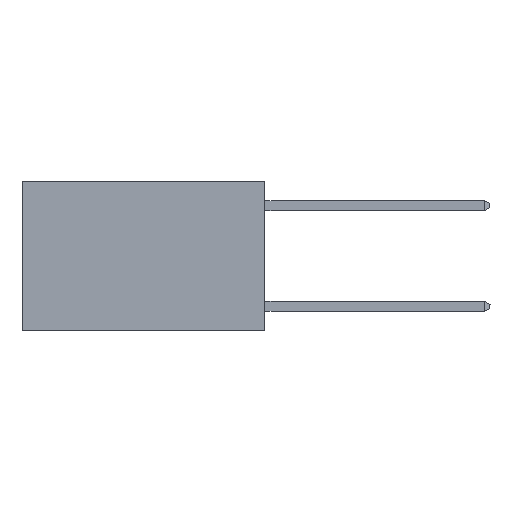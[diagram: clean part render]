
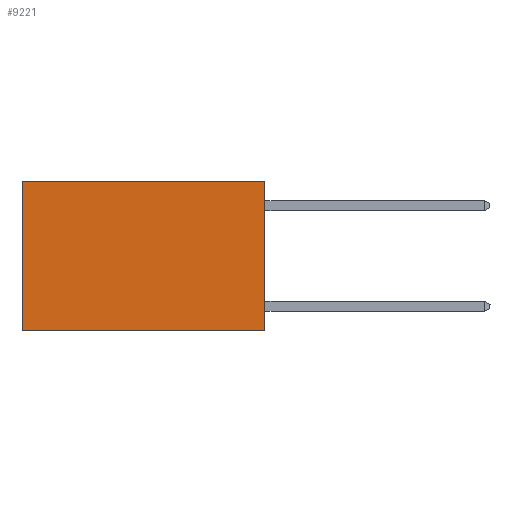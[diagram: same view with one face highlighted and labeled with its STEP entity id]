
A CAD part, left-side view. The second image highlights one B-rep face of the part: STEP entity #9221.
In plain terms, the highlighted planar face has unit normal (-1, 0, 0).
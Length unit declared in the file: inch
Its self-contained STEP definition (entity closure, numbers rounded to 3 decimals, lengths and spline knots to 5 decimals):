
#111 = CARTESIAN_POINT ( 'NONE',  ( 0.2625, 0., 0. ) ) ;
#2116 = VERTEX_POINT ( 'NONE', #5560 ) ;
#2221 = DIRECTION ( 'NONE',  ( 0., 1., 0. ) ) ;
#2553 = VECTOR ( 'NONE', #11673, 39.37008 ) ;
#3550 = ORIENTED_EDGE ( 'NONE', *, *, #9864, .T. ) ;
#4409 = CARTESIAN_POINT ( 'NONE',  ( 0.2625, 0.6, 0. ) ) ;
#4678 = EDGE_LOOP ( 'NONE', ( #14008, #14147, #18391, #3550 ) ) ;
#5560 = CARTESIAN_POINT ( 'NONE',  ( 0.2625, 0., 0. ) ) ;
#5922 = VERTEX_POINT ( 'NONE', #13095 ) ;
#6755 = EDGE_CURVE ( 'NONE', #5922, #15487, #7392, .T. ) ;
#6870 = LINE ( 'NONE', #23377, #11101 ) ;
#7136 = EDGE_CURVE ( 'NONE', #19478, #15487, #17420, .T. ) ;
#7240 = CARTESIAN_POINT ( 'NONE',  ( 0.2625, 0., 0. ) ) ;
#7392 = LINE ( 'NONE', #4409, #2553 ) ;
#7691 = VECTOR ( 'NONE', #2221, 39.37008 ) ;
#7881 = FACE_OUTER_BOUND ( 'NONE', #4678, .T. ) ;
#8148 = VECTOR ( 'NONE', #11087, 39.37008 ) ;
#8854 = DIRECTION ( 'NONE',  ( 0., 0., -1. ) ) ;
#9062 = DIRECTION ( 'NONE',  ( 1., 0., 0. ) ) ;
#9221 = ADVANCED_FACE ( 'NONE', ( #7881 ), #18153, .F. ) ;
#9631 = CARTESIAN_POINT ( 'NONE',  ( 0.2625, 0., -0.37 ) ) ;
#9864 = EDGE_CURVE ( 'NONE', #2116, #5922, #13576, .T. ) ;
#11087 = DIRECTION ( 'NONE',  ( 0., 1., 0. ) ) ;
#11101 = VECTOR ( 'NONE', #8854, 39.37008 ) ;
#11673 = DIRECTION ( 'NONE',  ( 0., 0., -1. ) ) ;
#13095 = CARTESIAN_POINT ( 'NONE',  ( 0.2625, 0.6, 0. ) ) ;
#13576 = LINE ( 'NONE', #111, #8148 ) ;
#14008 = ORIENTED_EDGE ( 'NONE', *, *, #6755, .T. ) ;
#14016 = CARTESIAN_POINT ( 'NONE',  ( 0.2625, 0.6, -0.37 ) ) ;
#14147 = ORIENTED_EDGE ( 'NONE', *, *, #7136, .F. ) ;
#14267 = EDGE_CURVE ( 'NONE', #2116, #19478, #6870, .T. ) ;
#15487 = VERTEX_POINT ( 'NONE', #14016 ) ;
#16809 = CARTESIAN_POINT ( 'NONE',  ( 0.2625, 0., -0.37 ) ) ;
#17420 = LINE ( 'NONE', #16809, #7691 ) ;
#18153 = PLANE ( 'NONE',  #23127 ) ;
#18391 = ORIENTED_EDGE ( 'NONE', *, *, #14267, .F. ) ;
#19478 = VERTEX_POINT ( 'NONE', #9631 ) ;
#21802 = DIRECTION ( 'NONE',  ( 0., 0., -1. ) ) ;
#23127 = AXIS2_PLACEMENT_3D ( 'NONE', #7240, #9062, #21802 ) ;
#23377 = CARTESIAN_POINT ( 'NONE',  ( 0.2625, 0., 0. ) ) ;
